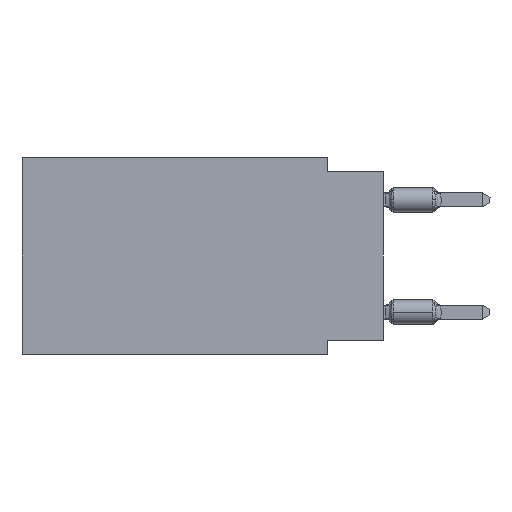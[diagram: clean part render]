
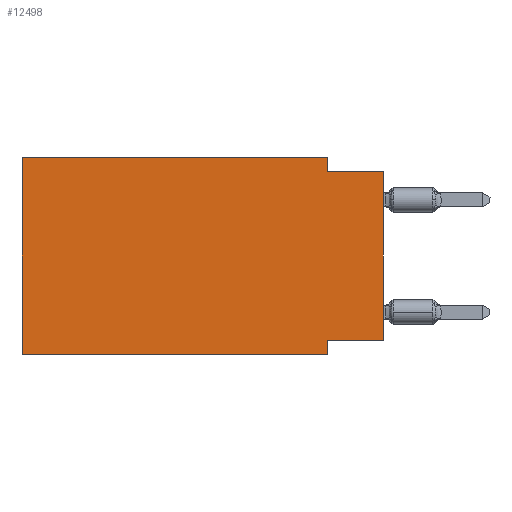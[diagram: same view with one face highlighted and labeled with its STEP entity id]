
A CAD part, left-side view. The second image highlights one B-rep face of the part: STEP entity #12498.
In plain terms, the highlighted planar face has unit normal (-1, 0, 0).
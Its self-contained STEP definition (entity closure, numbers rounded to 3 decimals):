
#372 = VECTOR ( 'NONE', #11204, 1000. ) ;
#503 = VECTOR ( 'NONE', #11100, 1000. ) ;
#883 = LINE ( 'NONE', #2684, #9929 ) ;
#904 = DIRECTION ( 'NONE',  ( 0., -1., 0. ) ) ;
#1043 = VECTOR ( 'NONE', #904, 1000. ) ;
#1286 = DIRECTION ( 'NONE',  ( 1., 0., 0. ) ) ;
#1292 = ORIENTED_EDGE ( 'NONE', *, *, #13086, .F. ) ;
#1301 = EDGE_CURVE ( 'NONE', #7398, #3766, #6668, .T. ) ;
#1394 = DIRECTION ( 'NONE',  ( 0., 1., 0. ) ) ;
#2282 = CARTESIAN_POINT ( 'NONE',  ( 0., 16.383, 0. ) ) ;
#2365 = CARTESIAN_POINT ( 'NONE',  ( 0., 0., -0.635 ) ) ;
#2668 = VECTOR ( 'NONE', #4346, 1000. ) ;
#2684 = CARTESIAN_POINT ( 'NONE',  ( 0., 2.54, -8.89 ) ) ;
#3092 = CARTESIAN_POINT ( 'NONE',  ( 0., 0., -0.635 ) ) ;
#3766 = VERTEX_POINT ( 'NONE', #5005 ) ;
#3780 = VERTEX_POINT ( 'NONE', #12523 ) ;
#4346 = DIRECTION ( 'NONE',  ( 0., -1., 0. ) ) ;
#4548 = CARTESIAN_POINT ( 'NONE',  ( 0., 0., -8.255 ) ) ;
#4623 = LINE ( 'NONE', #8829, #1043 ) ;
#4945 = VERTEX_POINT ( 'NONE', #13363 ) ;
#5005 = CARTESIAN_POINT ( 'NONE',  ( 0., 16.383, 0. ) ) ;
#5315 = VERTEX_POINT ( 'NONE', #10365 ) ;
#5380 = LINE ( 'NONE', #2365, #2668 ) ;
#5550 = ORIENTED_EDGE ( 'NONE', *, *, #1301, .F. ) ;
#5670 = EDGE_LOOP ( 'NONE', ( #11791, #8386, #7467, #1292, #5550, #5862, #11566, #6985 ) ) ;
#5824 = VERTEX_POINT ( 'NONE', #6206 ) ;
#5859 = AXIS2_PLACEMENT_3D ( 'NONE', #9613, #1286, #12857 ) ;
#5862 = ORIENTED_EDGE ( 'NONE', *, *, #13583, .T. ) ;
#5889 = CARTESIAN_POINT ( 'NONE',  ( 0., 0., 0. ) ) ;
#5907 = EDGE_CURVE ( 'NONE', #4945, #5315, #13104, .T. ) ;
#6089 = EDGE_CURVE ( 'NONE', #3780, #5824, #6891, .T. ) ;
#6206 = CARTESIAN_POINT ( 'NONE',  ( 0., 2.54, -0.635 ) ) ;
#6371 = PLANE ( 'NONE',  #5859 ) ;
#6668 = LINE ( 'NONE', #2282, #11700 ) ;
#6891 = LINE ( 'NONE', #8134, #503 ) ;
#6985 = ORIENTED_EDGE ( 'NONE', *, *, #5907, .F. ) ;
#7398 = VERTEX_POINT ( 'NONE', #13616 ) ;
#7467 = ORIENTED_EDGE ( 'NONE', *, *, #6089, .F. ) ;
#8134 = CARTESIAN_POINT ( 'NONE',  ( 0., 2.54, 0. ) ) ;
#8329 = DIRECTION ( 'NONE',  ( 0., -1., 0. ) ) ;
#8386 = ORIENTED_EDGE ( 'NONE', *, *, #9030, .F. ) ;
#8829 = CARTESIAN_POINT ( 'NONE',  ( 0., 16.383, 0. ) ) ;
#9030 = EDGE_CURVE ( 'NONE', #5824, #9962, #5380, .T. ) ;
#9232 = LINE ( 'NONE', #13441, #11840 ) ;
#9235 = CARTESIAN_POINT ( 'NONE',  ( 0., 2.54, -8.89 ) ) ;
#9426 = VERTEX_POINT ( 'NONE', #9235 ) ;
#9613 = CARTESIAN_POINT ( 'NONE',  ( 0., 16.383, 0. ) ) ;
#9717 = EDGE_CURVE ( 'NONE', #5315, #9426, #883, .T. ) ;
#9811 = LINE ( 'NONE', #5889, #372 ) ;
#9929 = VECTOR ( 'NONE', #10321, 1000. ) ;
#9962 = VERTEX_POINT ( 'NONE', #3092 ) ;
#10321 = DIRECTION ( 'NONE',  ( 0., 0., -1. ) ) ;
#10365 = CARTESIAN_POINT ( 'NONE',  ( 0., 2.54, -8.255 ) ) ;
#11100 = DIRECTION ( 'NONE',  ( 0., 0., -1. ) ) ;
#11204 = DIRECTION ( 'NONE',  ( 0., 0., 1. ) ) ;
#11566 = ORIENTED_EDGE ( 'NONE', *, *, #9717, .F. ) ;
#11700 = VECTOR ( 'NONE', #12689, 1000. ) ;
#11791 = ORIENTED_EDGE ( 'NONE', *, *, #12582, .T. ) ;
#11832 = FACE_OUTER_BOUND ( 'NONE', #5670, .T. ) ;
#11840 = VECTOR ( 'NONE', #8329, 1000. ) ;
#11957 = VECTOR ( 'NONE', #1394, 1000. ) ;
#12498 = ADVANCED_FACE ( 'NONE', ( #11832 ), #6371, .F. ) ;
#12523 = CARTESIAN_POINT ( 'NONE',  ( 0., 2.54, 0. ) ) ;
#12582 = EDGE_CURVE ( 'NONE', #4945, #9962, #9811, .T. ) ;
#12689 = DIRECTION ( 'NONE',  ( 0., 0., 1. ) ) ;
#12857 = DIRECTION ( 'NONE',  ( 0., 0., -1. ) ) ;
#13086 = EDGE_CURVE ( 'NONE', #3766, #3780, #4623, .T. ) ;
#13104 = LINE ( 'NONE', #4548, #11957 ) ;
#13363 = CARTESIAN_POINT ( 'NONE',  ( 0., 0., -8.255 ) ) ;
#13441 = CARTESIAN_POINT ( 'NONE',  ( 0., 16.383, -8.89 ) ) ;
#13583 = EDGE_CURVE ( 'NONE', #7398, #9426, #9232, .T. ) ;
#13616 = CARTESIAN_POINT ( 'NONE',  ( 0., 16.383, -8.89 ) ) ;
